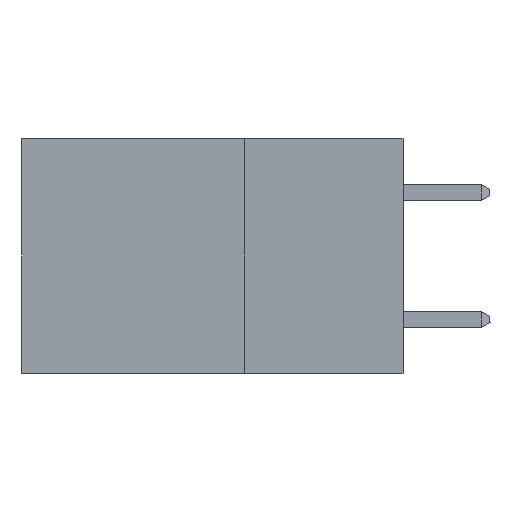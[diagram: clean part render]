
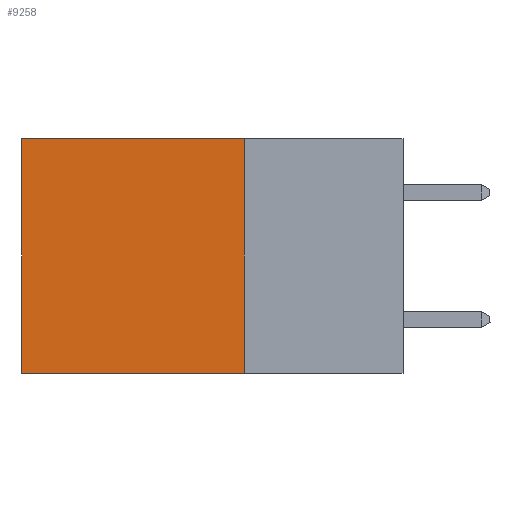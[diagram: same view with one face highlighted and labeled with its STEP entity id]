
A CAD part, left-side view. The second image highlights one B-rep face of the part: STEP entity #9258.
In plain terms, the highlighted planar face has unit normal (-1, 0, 0).
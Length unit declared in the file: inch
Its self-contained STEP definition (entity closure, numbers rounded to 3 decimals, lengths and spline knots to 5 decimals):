
#482 = LINE ( 'NONE', #6565, #1826 ) ;
#661 = CARTESIAN_POINT ( 'NONE',  ( 0.2875, 0.6, 0. ) ) ;
#789 = VECTOR ( 'NONE', #10381, 39.37008 ) ;
#1212 = EDGE_CURVE ( 'NONE', #15855, #20132, #17009, .T. ) ;
#1717 = CARTESIAN_POINT ( 'NONE',  ( 0.2875, 0.25, 0. ) ) ;
#1826 = VECTOR ( 'NONE', #15260, 39.37008 ) ;
#2088 = CARTESIAN_POINT ( 'NONE',  ( 0.2875, 0.25, -0.37 ) ) ;
#2129 = DIRECTION ( 'NONE',  ( 1., 0., 0. ) ) ;
#2671 = EDGE_CURVE ( 'NONE', #15855, #19029, #13819, .T. ) ;
#3642 = EDGE_CURVE ( 'NONE', #20132, #11258, #482, .T. ) ;
#3753 = FACE_OUTER_BOUND ( 'NONE', #16654, .T. ) ;
#4755 = VECTOR ( 'NONE', #9650, 39.37008 ) ;
#5333 = VECTOR ( 'NONE', #15736, 39.37008 ) ;
#6505 = PLANE ( 'NONE',  #9965 ) ;
#6565 = CARTESIAN_POINT ( 'NONE',  ( 0.2875, 0.6, 0. ) ) ;
#6605 = CARTESIAN_POINT ( 'NONE',  ( 0.2875, 0.25, 0. ) ) ;
#7661 = CARTESIAN_POINT ( 'NONE',  ( 0.2875, 0.6, -0.37 ) ) ;
#8046 = ORIENTED_EDGE ( 'NONE', *, *, #8934, .F. ) ;
#8934 = EDGE_CURVE ( 'NONE', #19029, #11258, #12023, .T. ) ;
#9258 = ADVANCED_FACE ( 'NONE', ( #3753 ), #6505, .F. ) ;
#9295 = ORIENTED_EDGE ( 'NONE', *, *, #2671, .F. ) ;
#9650 = DIRECTION ( 'NONE',  ( 0., 0., -1. ) ) ;
#9965 = AXIS2_PLACEMENT_3D ( 'NONE', #1717, #2129, #20430 ) ;
#10371 = CARTESIAN_POINT ( 'NONE',  ( 0.2875, 0.25, -0.37 ) ) ;
#10381 = DIRECTION ( 'NONE',  ( 0., 1., 0. ) ) ;
#11057 = ORIENTED_EDGE ( 'NONE', *, *, #3642, .T. ) ;
#11258 = VERTEX_POINT ( 'NONE', #7661 ) ;
#12023 = LINE ( 'NONE', #2088, #5333 ) ;
#13819 = LINE ( 'NONE', #14351, #4755 ) ;
#14351 = CARTESIAN_POINT ( 'NONE',  ( 0.2875, 0.25, 0. ) ) ;
#15260 = DIRECTION ( 'NONE',  ( 0., 0., -1. ) ) ;
#15736 = DIRECTION ( 'NONE',  ( 0., 1., 0. ) ) ;
#15855 = VERTEX_POINT ( 'NONE', #6605 ) ;
#16654 = EDGE_LOOP ( 'NONE', ( #11057, #8046, #9295, #18063 ) ) ;
#17009 = LINE ( 'NONE', #20532, #789 ) ;
#18063 = ORIENTED_EDGE ( 'NONE', *, *, #1212, .T. ) ;
#19029 = VERTEX_POINT ( 'NONE', #10371 ) ;
#20132 = VERTEX_POINT ( 'NONE', #661 ) ;
#20430 = DIRECTION ( 'NONE',  ( 0., 0., -1. ) ) ;
#20532 = CARTESIAN_POINT ( 'NONE',  ( 0.2875, 0.25, 0. ) ) ;
